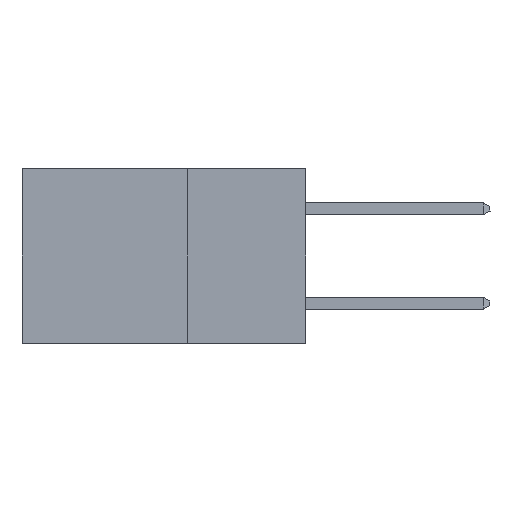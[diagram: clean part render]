
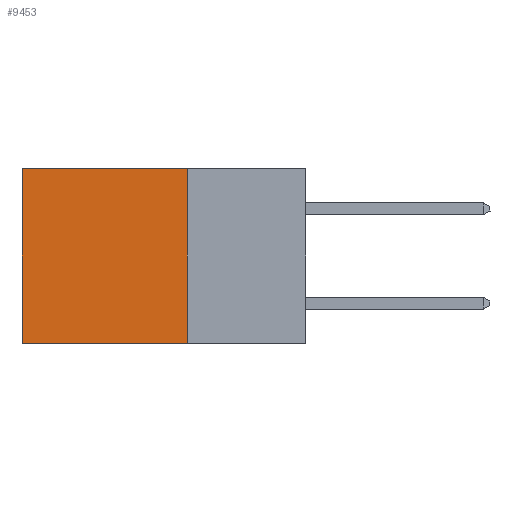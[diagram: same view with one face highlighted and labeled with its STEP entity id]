
A CAD part, left-side view. The second image highlights one B-rep face of the part: STEP entity #9453.
In plain terms, the highlighted planar face has unit normal (-1, 0, 0).
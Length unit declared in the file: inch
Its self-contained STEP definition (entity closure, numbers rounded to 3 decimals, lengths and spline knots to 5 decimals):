
#112 = CARTESIAN_POINT ( 'NONE',  ( 0.298, 0.25, 0. ) ) ;
#491 = FACE_OUTER_BOUND ( 'NONE', #3765, .T. ) ;
#1512 = VERTEX_POINT ( 'NONE', #112 ) ;
#1693 = VERTEX_POINT ( 'NONE', #11081 ) ;
#2246 = LINE ( 'NONE', #7464, #5768 ) ;
#2247 = DIRECTION ( 'NONE',  ( 0., 0., -1. ) ) ;
#2335 = AXIS2_PLACEMENT_3D ( 'NONE', #6500, #8125, #10905 ) ;
#2498 = DIRECTION ( 'NONE',  ( 0., 1., 0. ) ) ;
#2711 = ORIENTED_EDGE ( 'NONE', *, *, #6230, .T. ) ;
#2990 = ORIENTED_EDGE ( 'NONE', *, *, #4323, .F. ) ;
#3216 = DIRECTION ( 'NONE',  ( 0., 1., 0. ) ) ;
#3765 = EDGE_LOOP ( 'NONE', ( #7389, #4483, #2990, #2711 ) ) ;
#4034 = CARTESIAN_POINT ( 'NONE',  ( 0.298, 0.25, -0.37 ) ) ;
#4260 = VERTEX_POINT ( 'NONE', #4762 ) ;
#4323 = EDGE_CURVE ( 'NONE', #1512, #1693, #6750, .T. ) ;
#4483 = ORIENTED_EDGE ( 'NONE', *, *, #9980, .F. ) ;
#4762 = CARTESIAN_POINT ( 'NONE',  ( 0.298, 0.6, 0. ) ) ;
#4970 = CARTESIAN_POINT ( 'NONE',  ( 0.298, 0.6, -0.37 ) ) ;
#5322 = LINE ( 'NONE', #11171, #9060 ) ;
#5768 = VECTOR ( 'NONE', #2247, 39.37008 ) ;
#6230 = EDGE_CURVE ( 'NONE', #1512, #4260, #5322, .T. ) ;
#6500 = CARTESIAN_POINT ( 'NONE',  ( 0.298, 0.25, 0. ) ) ;
#6750 = LINE ( 'NONE', #8157, #9609 ) ;
#7088 = VERTEX_POINT ( 'NONE', #4970 ) ;
#7389 = ORIENTED_EDGE ( 'NONE', *, *, #11201, .T. ) ;
#7464 = CARTESIAN_POINT ( 'NONE',  ( 0.298, 0.6, 0. ) ) ;
#8125 = DIRECTION ( 'NONE',  ( 1., 0., 0. ) ) ;
#8151 = DIRECTION ( 'NONE',  ( 0., 0., -1. ) ) ;
#8157 = CARTESIAN_POINT ( 'NONE',  ( 0.298, 0.25, 0. ) ) ;
#8186 = PLANE ( 'NONE',  #2335 ) ;
#9060 = VECTOR ( 'NONE', #2498, 39.37008 ) ;
#9453 = ADVANCED_FACE ( 'NONE', ( #491 ), #8186, .F. ) ;
#9609 = VECTOR ( 'NONE', #8151, 39.37008 ) ;
#9980 = EDGE_CURVE ( 'NONE', #1693, #7088, #10448, .T. ) ;
#10448 = LINE ( 'NONE', #4034, #10570 ) ;
#10570 = VECTOR ( 'NONE', #3216, 39.37008 ) ;
#10905 = DIRECTION ( 'NONE',  ( 0., 0., -1. ) ) ;
#11081 = CARTESIAN_POINT ( 'NONE',  ( 0.298, 0.25, -0.37 ) ) ;
#11171 = CARTESIAN_POINT ( 'NONE',  ( 0.298, 0.25, 0. ) ) ;
#11201 = EDGE_CURVE ( 'NONE', #4260, #7088, #2246, .T. ) ;
